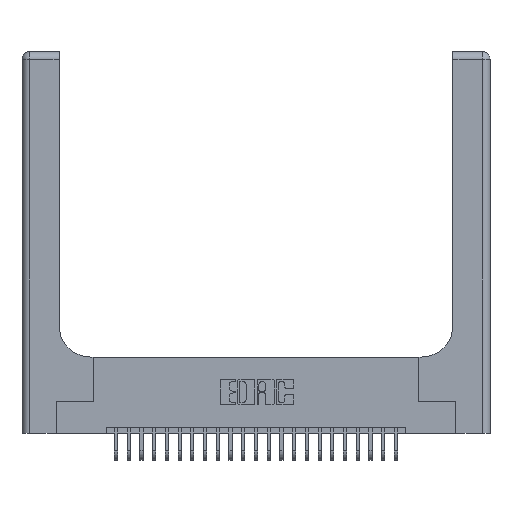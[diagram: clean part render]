
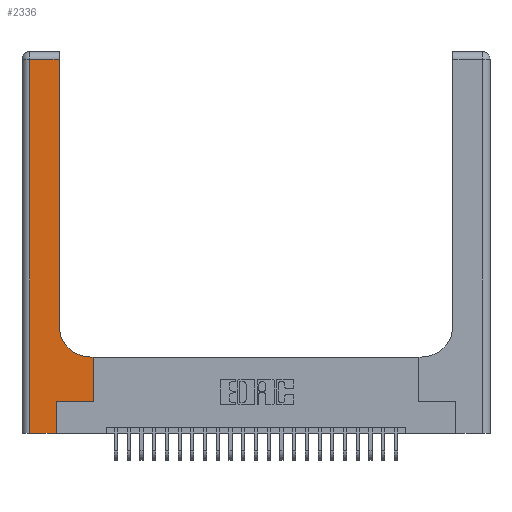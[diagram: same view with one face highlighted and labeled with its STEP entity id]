
A CAD part, top view. The second image highlights one B-rep face of the part: STEP entity #2336.
In plain terms, the highlighted planar face has unit normal (0, 0, 1).
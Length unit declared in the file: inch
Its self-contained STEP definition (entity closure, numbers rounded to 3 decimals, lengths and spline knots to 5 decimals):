
#166 = ORIENTED_EDGE ( 'NONE', *, *, #15120, .T. ) ;
#287 = CARTESIAN_POINT ( 'NONE',  ( 0.5415, 0.85, 0.37 ) ) ;
#614 = EDGE_CURVE ( 'NONE', #19628, #12212, #24317, .T. ) ;
#686 = CARTESIAN_POINT ( 'NONE',  ( 0.269, 0., 0.37 ) ) ;
#1780 = ORIENTED_EDGE ( 'NONE', *, *, #5930, .T. ) ;
#2060 = LINE ( 'NONE', #13204, #16909 ) ;
#2226 = EDGE_CURVE ( 'NONE', #24916, #16083, #8651, .T. ) ;
#2336 = ADVANCED_FACE ( 'NONE', ( #5361 ), #8462, .F. ) ;
#2882 = CARTESIAN_POINT ( 'NONE',  ( 0., 0., 0.37 ) ) ;
#3398 = VECTOR ( 'NONE', #10740, 39.37008 ) ;
#4391 = LINE ( 'NONE', #14704, #9352 ) ;
#4897 = VECTOR ( 'NONE', #11112, 39.37008 ) ;
#5361 = FACE_OUTER_BOUND ( 'NONE', #25893, .T. ) ;
#5401 = CARTESIAN_POINT ( 'NONE',  ( 0.5585, 0.25, 0.37 ) ) ;
#5597 = EDGE_CURVE ( 'NONE', #12212, #6294, #21369, .T. ) ;
#5930 = EDGE_CURVE ( 'NONE', #16083, #9923, #4391, .T. ) ;
#5942 = ORIENTED_EDGE ( 'NONE', *, *, #21685, .T. ) ;
#6294 = VERTEX_POINT ( 'NONE', #17867 ) ;
#6474 = VECTOR ( 'NONE', #25441, 39.37008 ) ;
#7052 = ORIENTED_EDGE ( 'NONE', *, *, #5597, .T. ) ;
#7343 = DIRECTION ( 'NONE',  ( 0., 1., 0. ) ) ;
#7409 = CIRCLE ( 'NONE', #25547, 0.25 ) ;
#7777 = ORIENTED_EDGE ( 'NONE', *, *, #16917, .T. ) ;
#7785 = VECTOR ( 'NONE', #15624, 39.37008 ) ;
#8290 = DIRECTION ( 'NONE',  ( -1., 0., 0. ) ) ;
#8378 = DIRECTION ( 'NONE',  ( 0., 0., -1. ) ) ;
#8462 = PLANE ( 'NONE',  #24136 ) ;
#8651 = LINE ( 'NONE', #2882, #3398 ) ;
#9352 = VECTOR ( 'NONE', #16843, 39.37008 ) ;
#9365 = CARTESIAN_POINT ( 'NONE',  ( 0.5585, 0.25, 0.37 ) ) ;
#9923 = VERTEX_POINT ( 'NONE', #16222 ) ;
#10472 = EDGE_CURVE ( 'NONE', #26581, #22632, #11071, .T. ) ;
#10740 = DIRECTION ( 'NONE',  ( 1., 0., 0. ) ) ;
#11071 = LINE ( 'NONE', #5401, #26357 ) ;
#11112 = DIRECTION ( 'NONE',  ( 0., -1., 0. ) ) ;
#11438 = VERTEX_POINT ( 'NONE', #18409 ) ;
#12212 = VERTEX_POINT ( 'NONE', #18400 ) ;
#12293 = DIRECTION ( 'NONE',  ( 1., 0., 0. ) ) ;
#13204 = CARTESIAN_POINT ( 'NONE',  ( 0.2915, 0.6, 0.37 ) ) ;
#14090 = ORIENTED_EDGE ( 'NONE', *, *, #10472, .T. ) ;
#14511 = CARTESIAN_POINT ( 'NONE',  ( 0., 3., 0.37 ) ) ;
#14704 = CARTESIAN_POINT ( 'NONE',  ( 0.269, 0., 0.37 ) ) ;
#15120 = EDGE_CURVE ( 'NONE', #6294, #24916, #21445, .T. ) ;
#15405 = DIRECTION ( 'NONE',  ( -1., 0., 0. ) ) ;
#15624 = DIRECTION ( 'NONE',  ( 0., 1., 0. ) ) ;
#16083 = VERTEX_POINT ( 'NONE', #686 ) ;
#16222 = CARTESIAN_POINT ( 'NONE',  ( 0.269, 0.25, 0.37 ) ) ;
#16424 = CARTESIAN_POINT ( 'NONE',  ( 0., 2.94, 0.37 ) ) ;
#16843 = DIRECTION ( 'NONE',  ( 0., 1., 0. ) ) ;
#16909 = VECTOR ( 'NONE', #15405, 39.37008 ) ;
#16917 = EDGE_CURVE ( 'NONE', #9923, #26581, #24009, .T. ) ;
#17867 = CARTESIAN_POINT ( 'NONE',  ( 0.06, 2.94, 0.37 ) ) ;
#18219 = EDGE_CURVE ( 'NONE', #11438, #19628, #7409, .T. ) ;
#18400 = CARTESIAN_POINT ( 'NONE',  ( 0.2915, 2.94, 0.37 ) ) ;
#18409 = CARTESIAN_POINT ( 'NONE',  ( 0.5415, 0.6, 0.37 ) ) ;
#19193 = DIRECTION ( 'NONE',  ( 1., 0., 0. ) ) ;
#19628 = VERTEX_POINT ( 'NONE', #22094 ) ;
#19815 = CARTESIAN_POINT ( 'NONE',  ( 0.06, 3., 0.37 ) ) ;
#20083 = CARTESIAN_POINT ( 'NONE',  ( 0.5585, 0.6, 0.37 ) ) ;
#21369 = LINE ( 'NONE', #16424, #6474 ) ;
#21445 = LINE ( 'NONE', #19815, #4897 ) ;
#21685 = EDGE_CURVE ( 'NONE', #22632, #11438, #2060, .T. ) ;
#22094 = CARTESIAN_POINT ( 'NONE',  ( 0.2915, 0.85, 0.37 ) ) ;
#22297 = CARTESIAN_POINT ( 'NONE',  ( 0.06, 0., 0.37 ) ) ;
#22632 = VERTEX_POINT ( 'NONE', #20083 ) ;
#22685 = VECTOR ( 'NONE', #12293, 39.37008 ) ;
#23442 = DIRECTION ( 'NONE',  ( 0., 0., -1. ) ) ;
#23768 = ORIENTED_EDGE ( 'NONE', *, *, #18219, .T. ) ;
#23990 = ORIENTED_EDGE ( 'NONE', *, *, #2226, .T. ) ;
#24009 = LINE ( 'NONE', #25083, #22685 ) ;
#24136 = AXIS2_PLACEMENT_3D ( 'NONE', #14511, #8378, #8290 ) ;
#24317 = LINE ( 'NONE', #26240, #7785 ) ;
#24916 = VERTEX_POINT ( 'NONE', #22297 ) ;
#25083 = CARTESIAN_POINT ( 'NONE',  ( 0.269, 0.25, 0.37 ) ) ;
#25441 = DIRECTION ( 'NONE',  ( -1., 0., 0. ) ) ;
#25547 = AXIS2_PLACEMENT_3D ( 'NONE', #287, #23442, #19193 ) ;
#25893 = EDGE_LOOP ( 'NONE', ( #27022, #7052, #166, #23990, #1780, #7777, #14090, #5942, #23768 ) ) ;
#26240 = CARTESIAN_POINT ( 'NONE',  ( 0.2915, 3., 0.37 ) ) ;
#26357 = VECTOR ( 'NONE', #7343, 39.37008 ) ;
#26581 = VERTEX_POINT ( 'NONE', #9365 ) ;
#27022 = ORIENTED_EDGE ( 'NONE', *, *, #614, .T. ) ;
